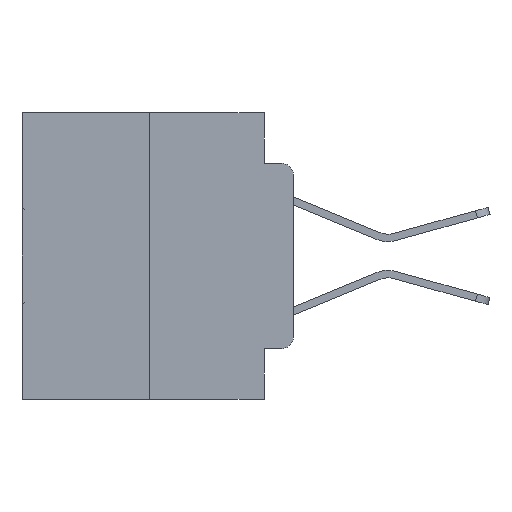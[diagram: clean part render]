
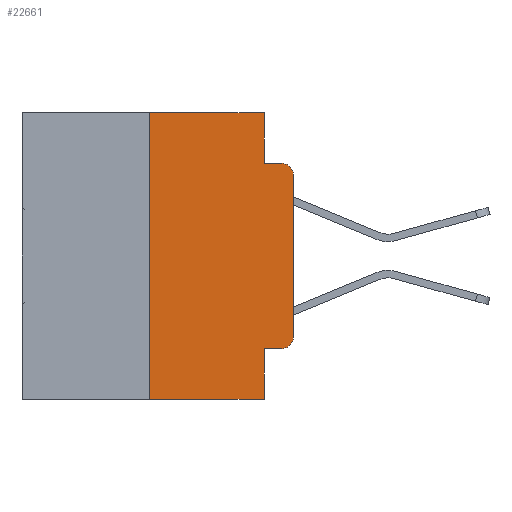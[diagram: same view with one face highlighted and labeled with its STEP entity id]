
A CAD part, left-side view. The second image highlights one B-rep face of the part: STEP entity #22661.
In plain terms, the highlighted planar face has unit normal (-1, 0, 0).
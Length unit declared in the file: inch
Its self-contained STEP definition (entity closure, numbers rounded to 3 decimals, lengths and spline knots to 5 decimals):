
#446 = ORIENTED_EDGE ( 'NONE', *, *, #28759, .F. ) ;
#701 = CARTESIAN_POINT ( 'NONE',  ( 0., 0., -0.1085 ) ) ;
#1559 = EDGE_CURVE ( 'NONE', #27159, #12849, #2333, .T. ) ;
#1877 = VECTOR ( 'NONE', #5140, 39.37008 ) ;
#2034 = VERTEX_POINT ( 'NONE', #12778 ) ;
#2072 = CARTESIAN_POINT ( 'NONE',  ( 0., 0., 0. ) ) ;
#2333 = CIRCLE ( 'NONE', #23564, 0.02 ) ;
#2624 = CARTESIAN_POINT ( 'NONE',  ( 0., 0.051, 0. ) ) ;
#2771 = LINE ( 'NONE', #2072, #16018 ) ;
#3216 = CARTESIAN_POINT ( 'NONE',  ( 0., 0.051, -0.4115 ) ) ;
#3470 = DIRECTION ( 'NONE',  ( 0., 0., -1. ) ) ;
#3886 = VERTEX_POINT ( 'NONE', #24519 ) ;
#4028 = ORIENTED_EDGE ( 'NONE', *, *, #6627, .T. ) ;
#4305 = FACE_OUTER_BOUND ( 'NONE', #31681, .T. ) ;
#5036 = VECTOR ( 'NONE', #21547, 39.37008 ) ;
#5140 = DIRECTION ( 'NONE',  ( 0., 0., -1. ) ) ;
#5593 = ORIENTED_EDGE ( 'NONE', *, *, #1559, .T. ) ;
#5663 = DIRECTION ( 'NONE',  ( 0., 0., -1. ) ) ;
#5727 = CARTESIAN_POINT ( 'NONE',  ( 0., 0., -0.3915 ) ) ;
#6627 = EDGE_CURVE ( 'NONE', #28296, #27159, #2771, .T. ) ;
#6767 = CIRCLE ( 'NONE', #21667, 0.02 ) ;
#7053 = EDGE_CURVE ( 'NONE', #16589, #21550, #28315, .T. ) ;
#8378 = CARTESIAN_POINT ( 'NONE',  ( 0., 0.051, 0. ) ) ;
#8510 = EDGE_CURVE ( 'NONE', #3886, #8731, #32057, .T. ) ;
#8666 = PLANE ( 'NONE',  #20676 ) ;
#8695 = CARTESIAN_POINT ( 'NONE',  ( 0., 0.473, -0.5 ) ) ;
#8731 = VERTEX_POINT ( 'NONE', #29647 ) ;
#9413 = VECTOR ( 'NONE', #26772, 39.37008 ) ;
#10401 = VERTEX_POINT ( 'NONE', #27728 ) ;
#11102 = VERTEX_POINT ( 'NONE', #3216 ) ;
#11180 = CARTESIAN_POINT ( 'NONE',  ( 0., 0.473, 0. ) ) ;
#11214 = DIRECTION ( 'NONE',  ( 0., -1., 0. ) ) ;
#12197 = ORIENTED_EDGE ( 'NONE', *, *, #32018, .F. ) ;
#12778 = CARTESIAN_POINT ( 'NONE',  ( 0., 0.02, -0.4115 ) ) ;
#12849 = VERTEX_POINT ( 'NONE', #18672 ) ;
#12965 = LINE ( 'NONE', #20375, #24646 ) ;
#13672 = DIRECTION ( 'NONE',  ( 1., 0., 0. ) ) ;
#14624 = DIRECTION ( 'NONE',  ( -1., 0., 0. ) ) ;
#15039 = VECTOR ( 'NONE', #3470, 39.37008 ) ;
#15206 = VECTOR ( 'NONE', #11214, 39.37008 ) ;
#15324 = ORIENTED_EDGE ( 'NONE', *, *, #8510, .F. ) ;
#16018 = VECTOR ( 'NONE', #19419, 39.37008 ) ;
#16589 = VERTEX_POINT ( 'NONE', #28184 ) ;
#18466 = ORIENTED_EDGE ( 'NONE', *, *, #23896, .F. ) ;
#18672 = CARTESIAN_POINT ( 'NONE',  ( 0., 0.02, -0.0885 ) ) ;
#18982 = CARTESIAN_POINT ( 'NONE',  ( 0., 0.051, -0.5 ) ) ;
#19419 = DIRECTION ( 'NONE',  ( 0., 0., 1. ) ) ;
#19678 = CARTESIAN_POINT ( 'NONE',  ( 0., 0.02, -0.1085 ) ) ;
#19762 = DIRECTION ( 'NONE',  ( 0., -1., 0. ) ) ;
#20375 = CARTESIAN_POINT ( 'NONE',  ( 0., 0.25, 0. ) ) ;
#20566 = EDGE_CURVE ( 'NONE', #2034, #28296, #6767, .T. ) ;
#20676 = AXIS2_PLACEMENT_3D ( 'NONE', #11180, #13672, #30878 ) ;
#21547 = DIRECTION ( 'NONE',  ( 0., -1., 0. ) ) ;
#21550 = VERTEX_POINT ( 'NONE', #18982 ) ;
#21641 = LINE ( 'NONE', #8378, #15039 ) ;
#21667 = AXIS2_PLACEMENT_3D ( 'NONE', #29354, #14624, #31796 ) ;
#21929 = ORIENTED_EDGE ( 'NONE', *, *, #25553, .F. ) ;
#22237 = EDGE_CURVE ( 'NONE', #11102, #2034, #29102, .T. ) ;
#22308 = LINE ( 'NONE', #31916, #29549 ) ;
#22661 = ADVANCED_FACE ( 'NONE', ( #4305 ), #8666, .F. ) ;
#22865 = DIRECTION ( 'NONE',  ( 0., 0., 1. ) ) ;
#23508 = ORIENTED_EDGE ( 'NONE', *, *, #7053, .T. ) ;
#23564 = AXIS2_PLACEMENT_3D ( 'NONE', #19678, #31449, #5663 ) ;
#23896 = EDGE_CURVE ( 'NONE', #11102, #21550, #21641, .T. ) ;
#24357 = CARTESIAN_POINT ( 'NONE',  ( 0., 0.051, -0.4115 ) ) ;
#24519 = CARTESIAN_POINT ( 'NONE',  ( 0., 0.25, 0. ) ) ;
#24646 = VECTOR ( 'NONE', #22865, 39.37008 ) ;
#25045 = ORIENTED_EDGE ( 'NONE', *, *, #22237, .T. ) ;
#25553 = EDGE_CURVE ( 'NONE', #16589, #3886, #12965, .T. ) ;
#26490 = CARTESIAN_POINT ( 'NONE',  ( 0., 0.473, 0. ) ) ;
#26772 = DIRECTION ( 'NONE',  ( 0., -1., 0. ) ) ;
#27159 = VERTEX_POINT ( 'NONE', #701 ) ;
#27728 = CARTESIAN_POINT ( 'NONE',  ( 0., 0.051, -0.0885 ) ) ;
#28184 = CARTESIAN_POINT ( 'NONE',  ( 0., 0.25, -0.5 ) ) ;
#28296 = VERTEX_POINT ( 'NONE', #5727 ) ;
#28315 = LINE ( 'NONE', #8695, #15206 ) ;
#28759 = EDGE_CURVE ( 'NONE', #8731, #10401, #29006, .T. ) ;
#29006 = LINE ( 'NONE', #2624, #1877 ) ;
#29102 = LINE ( 'NONE', #24357, #9413 ) ;
#29354 = CARTESIAN_POINT ( 'NONE',  ( 0., 0.02, -0.3915 ) ) ;
#29549 = VECTOR ( 'NONE', #19762, 39.37008 ) ;
#29647 = CARTESIAN_POINT ( 'NONE',  ( 0., 0.051, 0. ) ) ;
#30878 = DIRECTION ( 'NONE',  ( 0., 0., -1. ) ) ;
#31449 = DIRECTION ( 'NONE',  ( -1., 0., 0. ) ) ;
#31466 = ORIENTED_EDGE ( 'NONE', *, *, #20566, .T. ) ;
#31681 = EDGE_LOOP ( 'NONE', ( #4028, #5593, #12197, #446, #15324, #21929, #23508, #18466, #25045, #31466 ) ) ;
#31796 = DIRECTION ( 'NONE',  ( 0., 0., -1. ) ) ;
#31916 = CARTESIAN_POINT ( 'NONE',  ( 0., 0.051, -0.0885 ) ) ;
#32018 = EDGE_CURVE ( 'NONE', #10401, #12849, #22308, .T. ) ;
#32057 = LINE ( 'NONE', #26490, #5036 ) ;
